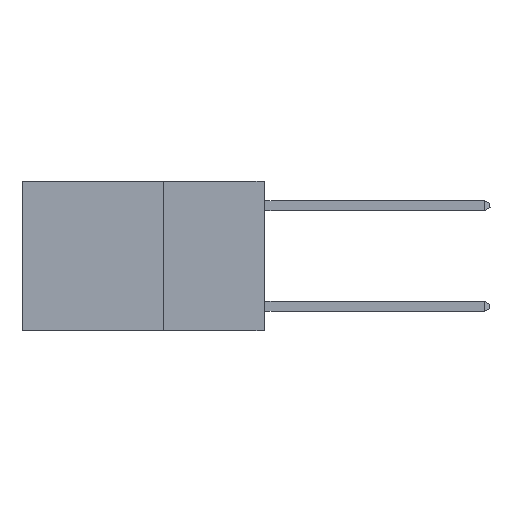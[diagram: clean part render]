
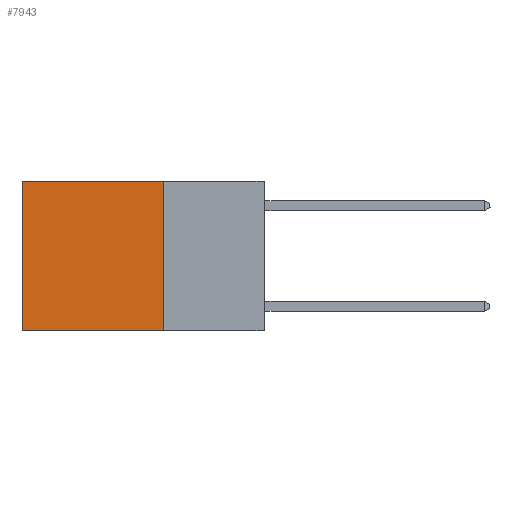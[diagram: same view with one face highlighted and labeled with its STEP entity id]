
A CAD part, left-side view. The second image highlights one B-rep face of the part: STEP entity #7943.
In plain terms, the highlighted planar face has unit normal (-1, 0, 0).
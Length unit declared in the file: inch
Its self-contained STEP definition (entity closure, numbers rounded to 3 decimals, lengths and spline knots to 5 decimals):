
#1104 = LINE ( 'NONE', #9040, #16768 ) ;
#2619 = ORIENTED_EDGE ( 'NONE', *, *, #11142, .T. ) ;
#3016 = FACE_OUTER_BOUND ( 'NONE', #7627, .T. ) ;
#3057 = CARTESIAN_POINT ( 'NONE',  ( 0.2625, 0.6, 0. ) ) ;
#3154 = DIRECTION ( 'NONE',  ( 0., 1., 0. ) ) ;
#3307 = PLANE ( 'NONE',  #24724 ) ;
#4551 = VECTOR ( 'NONE', #26695, 39.37008 ) ;
#4699 = VERTEX_POINT ( 'NONE', #16516 ) ;
#5684 = DIRECTION ( 'NONE',  ( 1., 0., 0. ) ) ;
#7486 = ORIENTED_EDGE ( 'NONE', *, *, #22983, .F. ) ;
#7627 = EDGE_LOOP ( 'NONE', ( #11621, #7486, #9570, #2619 ) ) ;
#7943 = ADVANCED_FACE ( 'NONE', ( #3016 ), #3307, .F. ) ;
#8156 = LINE ( 'NONE', #23078, #14596 ) ;
#8572 = LINE ( 'NONE', #3057, #4551 ) ;
#8714 = DIRECTION ( 'NONE',  ( 0., 1., 0. ) ) ;
#9040 = CARTESIAN_POINT ( 'NONE',  ( 0.2625, 0.25, 0. ) ) ;
#9117 = EDGE_CURVE ( 'NONE', #13732, #4699, #1104, .T. ) ;
#9570 = ORIENTED_EDGE ( 'NONE', *, *, #9117, .F. ) ;
#10436 = CARTESIAN_POINT ( 'NONE',  ( 0.2625, 0.25, 0. ) ) ;
#11142 = EDGE_CURVE ( 'NONE', #13732, #16153, #23297, .T. ) ;
#11621 = ORIENTED_EDGE ( 'NONE', *, *, #13294, .T. ) ;
#12184 = CARTESIAN_POINT ( 'NONE',  ( 0.2625, 0.25, 0. ) ) ;
#13284 = VERTEX_POINT ( 'NONE', #14862 ) ;
#13294 = EDGE_CURVE ( 'NONE', #16153, #13284, #8572, .T. ) ;
#13418 = CARTESIAN_POINT ( 'NONE',  ( 0.2625, 0.6, 0. ) ) ;
#13732 = VERTEX_POINT ( 'NONE', #27006 ) ;
#14596 = VECTOR ( 'NONE', #8714, 39.37008 ) ;
#14862 = CARTESIAN_POINT ( 'NONE',  ( 0.2625, 0.6, -0.37 ) ) ;
#16153 = VERTEX_POINT ( 'NONE', #13418 ) ;
#16516 = CARTESIAN_POINT ( 'NONE',  ( 0.2625, 0.25, -0.37 ) ) ;
#16768 = VECTOR ( 'NONE', #30692, 39.37008 ) ;
#22983 = EDGE_CURVE ( 'NONE', #4699, #13284, #8156, .T. ) ;
#23078 = CARTESIAN_POINT ( 'NONE',  ( 0.2625, 0.25, -0.37 ) ) ;
#23297 = LINE ( 'NONE', #12184, #25541 ) ;
#24724 = AXIS2_PLACEMENT_3D ( 'NONE', #10436, #5684, #27148 ) ;
#25541 = VECTOR ( 'NONE', #3154, 39.37008 ) ;
#26695 = DIRECTION ( 'NONE',  ( 0., 0., -1. ) ) ;
#27006 = CARTESIAN_POINT ( 'NONE',  ( 0.2625, 0.25, 0. ) ) ;
#27148 = DIRECTION ( 'NONE',  ( 0., 0., -1. ) ) ;
#30692 = DIRECTION ( 'NONE',  ( 0., 0., -1. ) ) ;
